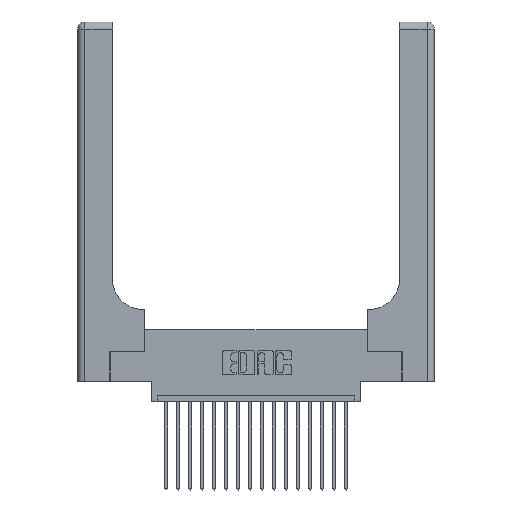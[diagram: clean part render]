
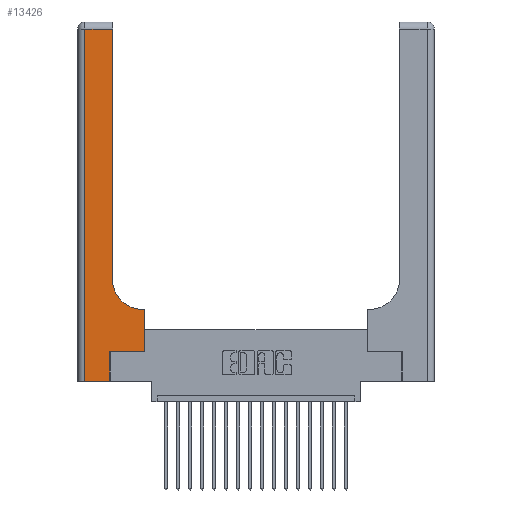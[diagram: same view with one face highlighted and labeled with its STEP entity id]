
A CAD part, top view. The second image highlights one B-rep face of the part: STEP entity #13426.
In plain terms, the highlighted planar face has unit normal (0, 0, 1).
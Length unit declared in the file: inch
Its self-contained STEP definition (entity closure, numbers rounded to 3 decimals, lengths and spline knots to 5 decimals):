
#75 = EDGE_CURVE ( 'NONE', #4230, #5688, #1475, .T. ) ;
#390 = EDGE_CURVE ( 'NONE', #6248, #4230, #20877, .T. ) ;
#1025 = ORIENTED_EDGE ( 'NONE', *, *, #6437, .T. ) ;
#1160 = ORIENTED_EDGE ( 'NONE', *, *, #15975, .T. ) ;
#1425 = VECTOR ( 'NONE', #10409, 39.37008 ) ;
#1475 = LINE ( 'NONE', #20606, #18631 ) ;
#1557 = DIRECTION ( 'NONE',  ( 0., 1., 0. ) ) ;
#1731 = ORIENTED_EDGE ( 'NONE', *, *, #9021, .T. ) ;
#1929 = CARTESIAN_POINT ( 'NONE',  ( 0.5415, 0.6, 0.37 ) ) ;
#1949 = CARTESIAN_POINT ( 'NONE',  ( 0.5585, 0.6, 0.37 ) ) ;
#1951 = AXIS2_PLACEMENT_3D ( 'NONE', #14594, #4880, #17582 ) ;
#2019 = CARTESIAN_POINT ( 'NONE',  ( 0.06, 2.94, 0.37 ) ) ;
#2885 = EDGE_CURVE ( 'NONE', #14469, #17948, #14404, .T. ) ;
#3194 = CARTESIAN_POINT ( 'NONE',  ( 0.269, 0.25, 0.37 ) ) ;
#4230 = VERTEX_POINT ( 'NONE', #11041 ) ;
#4690 = DIRECTION ( 'NONE',  ( 1., 0., 0. ) ) ;
#4766 = DIRECTION ( 'NONE',  ( 0., 0., -1. ) ) ;
#4880 = DIRECTION ( 'NONE',  ( 0., 0., -1. ) ) ;
#5684 = VERTEX_POINT ( 'NONE', #1949 ) ;
#5688 = VERTEX_POINT ( 'NONE', #2019 ) ;
#6108 = CARTESIAN_POINT ( 'NONE',  ( 0.5585, 0.25, 0.37 ) ) ;
#6248 = VERTEX_POINT ( 'NONE', #10061 ) ;
#6437 = EDGE_CURVE ( 'NONE', #8251, #8820, #14234, .T. ) ;
#6789 = DIRECTION ( 'NONE',  ( 1., 0., 0. ) ) ;
#6919 = LINE ( 'NONE', #11293, #17254 ) ;
#7668 = DIRECTION ( 'NONE',  ( -1., 0., 0. ) ) ;
#8068 = CARTESIAN_POINT ( 'NONE',  ( 0.2915, 0.6, 0.37 ) ) ;
#8244 = EDGE_CURVE ( 'NONE', #8432, #6248, #17154, .T. ) ;
#8251 = VERTEX_POINT ( 'NONE', #3194 ) ;
#8277 = CARTESIAN_POINT ( 'NONE',  ( 0.5415, 0.85, 0.37 ) ) ;
#8432 = VERTEX_POINT ( 'NONE', #1929 ) ;
#8579 = VECTOR ( 'NONE', #12213, 39.37008 ) ;
#8820 = VERTEX_POINT ( 'NONE', #6108 ) ;
#9021 = EDGE_CURVE ( 'NONE', #5684, #8432, #10849, .T. ) ;
#9357 = ORIENTED_EDGE ( 'NONE', *, *, #8244, .T. ) ;
#10061 = CARTESIAN_POINT ( 'NONE',  ( 0.2915, 0.85, 0.37 ) ) ;
#10409 = DIRECTION ( 'NONE',  ( 0., 1., 0. ) ) ;
#10748 = VECTOR ( 'NONE', #1557, 39.37008 ) ;
#10849 = LINE ( 'NONE', #8068, #14140 ) ;
#11041 = CARTESIAN_POINT ( 'NONE',  ( 0.2915, 2.94, 0.37 ) ) ;
#11062 = LINE ( 'NONE', #16731, #1425 ) ;
#11159 = ORIENTED_EDGE ( 'NONE', *, *, #16876, .T. ) ;
#11293 = CARTESIAN_POINT ( 'NONE',  ( 0.06, 3., 0.37 ) ) ;
#11444 = DIRECTION ( 'NONE',  ( 0., -1., 0. ) ) ;
#11477 = AXIS2_PLACEMENT_3D ( 'NONE', #8277, #4766, #4690 ) ;
#12213 = DIRECTION ( 'NONE',  ( 0., 1., 0. ) ) ;
#12560 = EDGE_CURVE ( 'NONE', #5688, #14469, #6919, .T. ) ;
#12895 = PLANE ( 'NONE',  #1951 ) ;
#13107 = DIRECTION ( 'NONE',  ( 1., 0., 0. ) ) ;
#13426 = ADVANCED_FACE ( 'NONE', ( #17987 ), #12895, .F. ) ;
#14140 = VECTOR ( 'NONE', #17854, 39.37008 ) ;
#14234 = LINE ( 'NONE', #16960, #20472 ) ;
#14280 = EDGE_LOOP ( 'NONE', ( #20366, #17736, #19165, #20330, #1160, #1025, #11159, #1731, #9357 ) ) ;
#14404 = LINE ( 'NONE', #19307, #18154 ) ;
#14469 = VERTEX_POINT ( 'NONE', #17296 ) ;
#14594 = CARTESIAN_POINT ( 'NONE',  ( 0., 3., 0.37 ) ) ;
#15975 = EDGE_CURVE ( 'NONE', #17948, #8251, #11062, .T. ) ;
#16055 = CARTESIAN_POINT ( 'NONE',  ( 0.5585, 0.25, 0.37 ) ) ;
#16731 = CARTESIAN_POINT ( 'NONE',  ( 0.269, 0., 0.37 ) ) ;
#16876 = EDGE_CURVE ( 'NONE', #8820, #5684, #17052, .T. ) ;
#16960 = CARTESIAN_POINT ( 'NONE',  ( 0.269, 0.25, 0.37 ) ) ;
#17052 = LINE ( 'NONE', #16055, #10748 ) ;
#17154 = CIRCLE ( 'NONE', #11477, 0.25 ) ;
#17254 = VECTOR ( 'NONE', #11444, 39.37008 ) ;
#17296 = CARTESIAN_POINT ( 'NONE',  ( 0.06, 0., 0.37 ) ) ;
#17582 = DIRECTION ( 'NONE',  ( -1., 0., 0. ) ) ;
#17736 = ORIENTED_EDGE ( 'NONE', *, *, #75, .T. ) ;
#17854 = DIRECTION ( 'NONE',  ( -1., 0., 0. ) ) ;
#17948 = VERTEX_POINT ( 'NONE', #18908 ) ;
#17987 = FACE_OUTER_BOUND ( 'NONE', #14280, .T. ) ;
#18154 = VECTOR ( 'NONE', #13107, 39.37008 ) ;
#18631 = VECTOR ( 'NONE', #7668, 39.37008 ) ;
#18645 = CARTESIAN_POINT ( 'NONE',  ( 0.2915, 3., 0.37 ) ) ;
#18908 = CARTESIAN_POINT ( 'NONE',  ( 0.269, 0., 0.37 ) ) ;
#19165 = ORIENTED_EDGE ( 'NONE', *, *, #12560, .T. ) ;
#19307 = CARTESIAN_POINT ( 'NONE',  ( 0., 0., 0.37 ) ) ;
#20330 = ORIENTED_EDGE ( 'NONE', *, *, #2885, .T. ) ;
#20366 = ORIENTED_EDGE ( 'NONE', *, *, #390, .T. ) ;
#20472 = VECTOR ( 'NONE', #6789, 39.37008 ) ;
#20606 = CARTESIAN_POINT ( 'NONE',  ( 0., 2.94, 0.37 ) ) ;
#20877 = LINE ( 'NONE', #18645, #8579 ) ;
